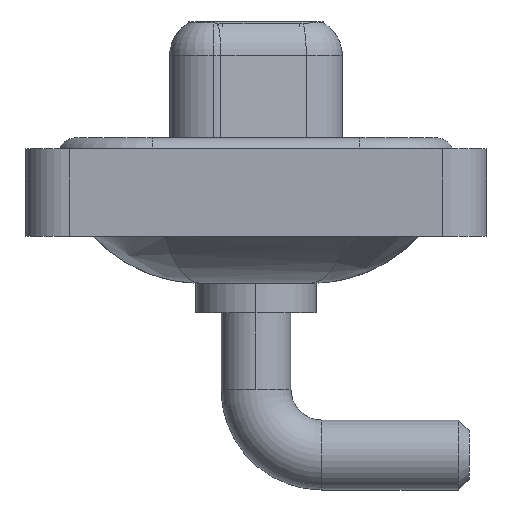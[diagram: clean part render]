
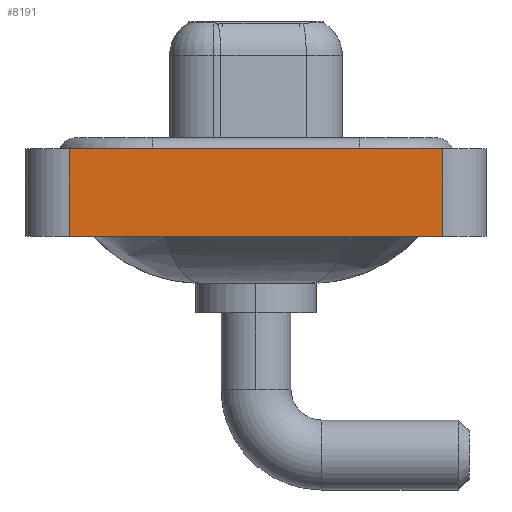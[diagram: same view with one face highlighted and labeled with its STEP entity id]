
A CAD part, left-side view. The second image highlights one B-rep face of the part: STEP entity #8191.
In plain terms, the highlighted planar face has unit normal (-1, 0, 0).
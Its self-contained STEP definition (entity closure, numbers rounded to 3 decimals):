
#229 = VECTOR ( 'NONE', #7147, 1000. ) ;
#892 = CARTESIAN_POINT ( 'NONE',  ( -7.3, -8.55, 0.4 ) ) ;
#1840 = DIRECTION ( 'NONE',  ( 0., -1., 0. ) ) ;
#2534 = ORIENTED_EDGE ( 'NONE', *, *, #6992, .T. ) ;
#2942 = CARTESIAN_POINT ( 'NONE',  ( -7.3, -8.55, -3.6 ) ) ;
#3554 = EDGE_LOOP ( 'NONE', ( #10265, #12739, #6640, #2534 ) ) ;
#3645 = VERTEX_POINT ( 'NONE', #9617 ) ;
#3686 = FACE_OUTER_BOUND ( 'NONE', #3554, .T. ) ;
#4820 = DIRECTION ( 'NONE',  ( 0., 0., 1. ) ) ;
#5368 = LINE ( 'NONE', #2942, #12890 ) ;
#5719 = CARTESIAN_POINT ( 'NONE',  ( -7.3, -8.55, -3.6 ) ) ;
#5868 = VECTOR ( 'NONE', #13370, 1000. ) ;
#6051 = VERTEX_POINT ( 'NONE', #892 ) ;
#6118 = CARTESIAN_POINT ( 'NONE',  ( -7.3, -8.55, -3.6 ) ) ;
#6282 = LINE ( 'NONE', #13376, #229 ) ;
#6640 = ORIENTED_EDGE ( 'NONE', *, *, #10658, .F. ) ;
#6992 = EDGE_CURVE ( 'NONE', #11722, #11103, #9279, .T. ) ;
#7147 = DIRECTION ( 'NONE',  ( 0., 0., 1. ) ) ;
#7758 = LINE ( 'NONE', #12687, #5868 ) ;
#8191 = ADVANCED_FACE ( 'NONE', ( #3686 ), #9754, .T. ) ;
#8458 = DIRECTION ( 'NONE',  ( -1., 0., 0. ) ) ;
#8504 = CARTESIAN_POINT ( 'NONE',  ( -7.3, 8.55, -3.6 ) ) ;
#9279 = LINE ( 'NONE', #5719, #15099 ) ;
#9617 = CARTESIAN_POINT ( 'NONE',  ( -7.3, 8.55, 0.4 ) ) ;
#9754 = PLANE ( 'NONE',  #12521 ) ;
#10265 = ORIENTED_EDGE ( 'NONE', *, *, #11397, .T. ) ;
#10658 = EDGE_CURVE ( 'NONE', #11722, #3645, #6282, .T. ) ;
#10703 = CARTESIAN_POINT ( 'NONE',  ( -7.3, -8.55, -3.6 ) ) ;
#11103 = VERTEX_POINT ( 'NONE', #10703 ) ;
#11397 = EDGE_CURVE ( 'NONE', #11103, #6051, #5368, .T. ) ;
#11722 = VERTEX_POINT ( 'NONE', #8504 ) ;
#12521 = AXIS2_PLACEMENT_3D ( 'NONE', #6118, #8458, #4820 ) ;
#12551 = DIRECTION ( 'NONE',  ( 0., 0., 1. ) ) ;
#12687 = CARTESIAN_POINT ( 'NONE',  ( -7.3, -8.55, 0.4 ) ) ;
#12739 = ORIENTED_EDGE ( 'NONE', *, *, #15204, .F. ) ;
#12890 = VECTOR ( 'NONE', #12551, 1000. ) ;
#13370 = DIRECTION ( 'NONE',  ( 0., -1., 0. ) ) ;
#13376 = CARTESIAN_POINT ( 'NONE',  ( -7.3, 8.55, -3.6 ) ) ;
#15099 = VECTOR ( 'NONE', #1840, 1000. ) ;
#15204 = EDGE_CURVE ( 'NONE', #3645, #6051, #7758, .T. ) ;
